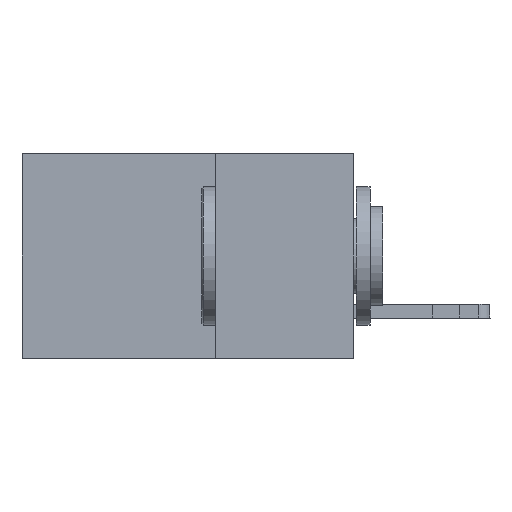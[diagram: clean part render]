
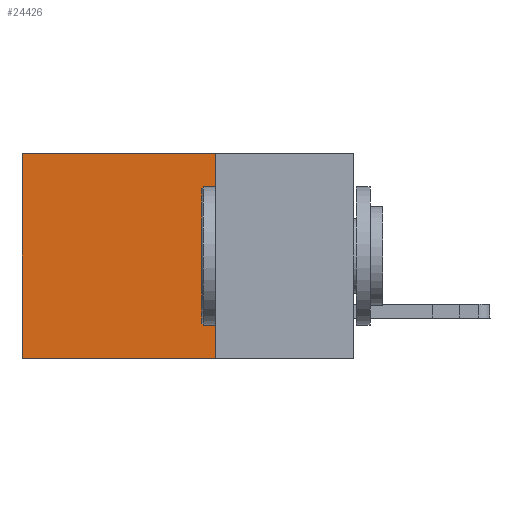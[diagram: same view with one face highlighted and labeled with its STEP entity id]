
A CAD part, left-side view. The second image highlights one B-rep face of the part: STEP entity #24426.
In plain terms, the highlighted planar face has unit normal (-1, 0, 0).
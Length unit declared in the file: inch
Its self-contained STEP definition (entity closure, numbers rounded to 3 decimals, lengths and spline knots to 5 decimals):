
#274 = FACE_OUTER_BOUND ( 'NONE', #17817, .T. ) ;
#2433 = PLANE ( 'NONE',  #27233 ) ;
#3719 = DIRECTION ( 'NONE',  ( 0., 0., -1. ) ) ;
#4518 = VERTEX_POINT ( 'NONE', #22122 ) ;
#6441 = EDGE_CURVE ( 'NONE', #26316, #18224, #23165, .T. ) ;
#7211 = VECTOR ( 'NONE', #19167, 39.37008 ) ;
#7336 = DIRECTION ( 'NONE',  ( 1., 0., 0. ) ) ;
#7459 = CARTESIAN_POINT ( 'NONE',  ( 0.2875, 0.25, 0. ) ) ;
#7957 = LINE ( 'NONE', #11821, #7211 ) ;
#9430 = VECTOR ( 'NONE', #3719, 39.37008 ) ;
#10123 = VECTOR ( 'NONE', #30979, 39.37008 ) ;
#10733 = ORIENTED_EDGE ( 'NONE', *, *, #24106, .T. ) ;
#11821 = CARTESIAN_POINT ( 'NONE',  ( 0.2875, 0.25, 0. ) ) ;
#12380 = DIRECTION ( 'NONE',  ( 0., 1., 0. ) ) ;
#15302 = VECTOR ( 'NONE', #12380, 39.37008 ) ;
#16395 = CARTESIAN_POINT ( 'NONE',  ( 0.2875, 0.25, 0. ) ) ;
#16855 = EDGE_CURVE ( 'NONE', #18224, #17815, #29035, .T. ) ;
#17815 = VERTEX_POINT ( 'NONE', #18919 ) ;
#17817 = EDGE_LOOP ( 'NONE', ( #10733, #24815, #18045, #28844 ) ) ;
#18045 = ORIENTED_EDGE ( 'NONE', *, *, #6441, .F. ) ;
#18224 = VERTEX_POINT ( 'NONE', #30502 ) ;
#18344 = CARTESIAN_POINT ( 'NONE',  ( 0.2875, 0.6, 0. ) ) ;
#18919 = CARTESIAN_POINT ( 'NONE',  ( 0.2875, 0.6, -0.37 ) ) ;
#19167 = DIRECTION ( 'NONE',  ( 0., 1., 0. ) ) ;
#21991 = CARTESIAN_POINT ( 'NONE',  ( 0.2875, 0.25, 0. ) ) ;
#22122 = CARTESIAN_POINT ( 'NONE',  ( 0.2875, 0.6, 0. ) ) ;
#22456 = LINE ( 'NONE', #18344, #9430 ) ;
#23165 = LINE ( 'NONE', #16395, #10123 ) ;
#23319 = EDGE_CURVE ( 'NONE', #26316, #4518, #7957, .T. ) ;
#24106 = EDGE_CURVE ( 'NONE', #4518, #17815, #22456, .T. ) ;
#24426 = ADVANCED_FACE ( 'NONE', ( #274 ), #2433, .F. ) ;
#24441 = DIRECTION ( 'NONE',  ( 0., 0., -1. ) ) ;
#24563 = CARTESIAN_POINT ( 'NONE',  ( 0.2875, 0.25, -0.37 ) ) ;
#24815 = ORIENTED_EDGE ( 'NONE', *, *, #16855, .F. ) ;
#26316 = VERTEX_POINT ( 'NONE', #7459 ) ;
#27233 = AXIS2_PLACEMENT_3D ( 'NONE', #21991, #7336, #24441 ) ;
#28844 = ORIENTED_EDGE ( 'NONE', *, *, #23319, .T. ) ;
#29035 = LINE ( 'NONE', #24563, #15302 ) ;
#30502 = CARTESIAN_POINT ( 'NONE',  ( 0.2875, 0.25, -0.37 ) ) ;
#30979 = DIRECTION ( 'NONE',  ( 0., 0., -1. ) ) ;
